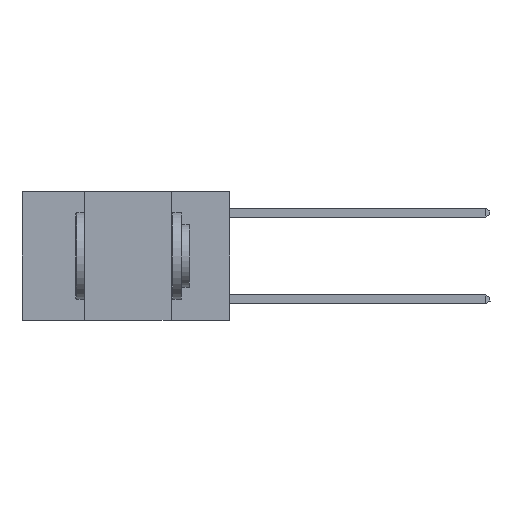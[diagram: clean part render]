
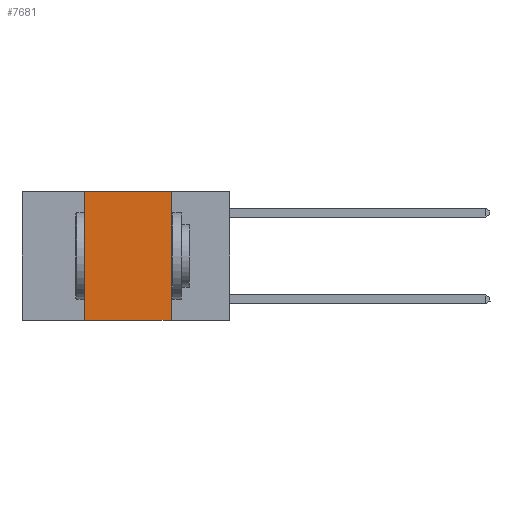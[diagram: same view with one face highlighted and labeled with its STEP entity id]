
A CAD part, left-side view. The second image highlights one B-rep face of the part: STEP entity #7681.
In plain terms, the highlighted planar face has unit normal (-1, 0, 0).
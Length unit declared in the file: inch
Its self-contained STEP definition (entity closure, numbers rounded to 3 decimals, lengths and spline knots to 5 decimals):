
#333 = CARTESIAN_POINT ( 'NONE',  ( 0., 0.42, 0. ) ) ;
#662 = EDGE_CURVE ( 'NONE', #8073, #2664, #7181, .T. ) ;
#725 = DIRECTION ( 'NONE',  ( 1., 0., 0. ) ) ;
#1760 = AXIS2_PLACEMENT_3D ( 'NONE', #12667, #725, #12742 ) ;
#2483 = EDGE_CURVE ( 'NONE', #6628, #8073, #21799, .T. ) ;
#2664 = VERTEX_POINT ( 'NONE', #14545 ) ;
#3740 = CARTESIAN_POINT ( 'NONE',  ( 0., 0.42, 0. ) ) ;
#4280 = ORIENTED_EDGE ( 'NONE', *, *, #16999, .T. ) ;
#4470 = LINE ( 'NONE', #3740, #21980 ) ;
#6628 = VERTEX_POINT ( 'NONE', #333 ) ;
#7181 = LINE ( 'NONE', #17700, #11753 ) ;
#7681 = ADVANCED_FACE ( 'NONE', ( #12413 ), #17768, .F. ) ;
#8073 = VERTEX_POINT ( 'NONE', #10176 ) ;
#8241 = EDGE_CURVE ( 'NONE', #20630, #6628, #4470, .T. ) ;
#9810 = LINE ( 'NONE', #11259, #17803 ) ;
#10176 = CARTESIAN_POINT ( 'NONE',  ( 0., 0.17, 0. ) ) ;
#10605 = DIRECTION ( 'NONE',  ( 0., 0., 1. ) ) ;
#10735 = DIRECTION ( 'NONE',  ( 0., -1., 0. ) ) ;
#11259 = CARTESIAN_POINT ( 'NONE',  ( 0., 0.6, -0.37 ) ) ;
#11753 = VECTOR ( 'NONE', #19081, 39.37008 ) ;
#12315 = ORIENTED_EDGE ( 'NONE', *, *, #2483, .F. ) ;
#12413 = FACE_OUTER_BOUND ( 'NONE', #20298, .T. ) ;
#12667 = CARTESIAN_POINT ( 'NONE',  ( 0., 0.6, 0. ) ) ;
#12742 = DIRECTION ( 'NONE',  ( 0., 0., -1. ) ) ;
#12864 = VECTOR ( 'NONE', #10735, 39.37008 ) ;
#14545 = CARTESIAN_POINT ( 'NONE',  ( 0., 0.17, -0.37 ) ) ;
#15234 = CARTESIAN_POINT ( 'NONE',  ( 0., 0.42, -0.37 ) ) ;
#16273 = ORIENTED_EDGE ( 'NONE', *, *, #662, .F. ) ;
#16380 = DIRECTION ( 'NONE',  ( 0., -1., 0. ) ) ;
#16999 = EDGE_CURVE ( 'NONE', #20630, #2664, #9810, .T. ) ;
#17700 = CARTESIAN_POINT ( 'NONE',  ( 0., 0.17, 0. ) ) ;
#17768 = PLANE ( 'NONE',  #1760 ) ;
#17803 = VECTOR ( 'NONE', #16380, 39.37008 ) ;
#19081 = DIRECTION ( 'NONE',  ( 0., 0., -1. ) ) ;
#20298 = EDGE_LOOP ( 'NONE', ( #16273, #12315, #21271, #4280 ) ) ;
#20630 = VERTEX_POINT ( 'NONE', #15234 ) ;
#20853 = CARTESIAN_POINT ( 'NONE',  ( 0., 0.6, 0. ) ) ;
#21271 = ORIENTED_EDGE ( 'NONE', *, *, #8241, .F. ) ;
#21799 = LINE ( 'NONE', #20853, #12864 ) ;
#21980 = VECTOR ( 'NONE', #10605, 39.37008 ) ;
